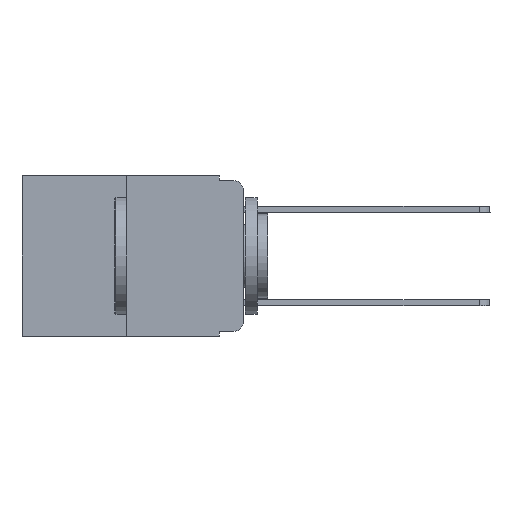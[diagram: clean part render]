
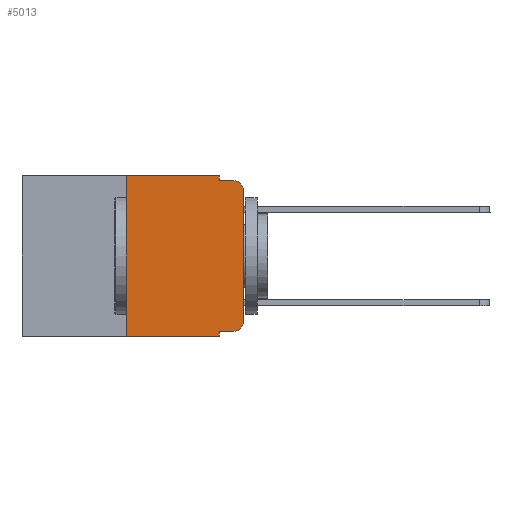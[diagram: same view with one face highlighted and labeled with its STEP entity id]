
A CAD part, left-side view. The second image highlights one B-rep face of the part: STEP entity #5013.
In plain terms, the highlighted planar face has unit normal (-1, 0, 0).
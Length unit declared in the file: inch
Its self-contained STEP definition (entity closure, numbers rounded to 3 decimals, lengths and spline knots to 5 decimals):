
#557 = VECTOR ( 'NONE', #19836, 39.37008 ) ;
#812 = VECTOR ( 'NONE', #2644, 39.37008 ) ;
#824 = VERTEX_POINT ( 'NONE', #6259 ) ;
#881 = EDGE_CURVE ( 'NONE', #18751, #15589, #11647, .T. ) ;
#998 = CARTESIAN_POINT ( 'NONE',  ( 0., 0.25, 0. ) ) ;
#1251 = PLANE ( 'NONE',  #21415 ) ;
#1456 = CARTESIAN_POINT ( 'NONE',  ( 0., 0.02, -0.333 ) ) ;
#1478 = EDGE_CURVE ( 'NONE', #9286, #5018, #22921, .T. ) ;
#2509 = ORIENTED_EDGE ( 'NONE', *, *, #4705, .F. ) ;
#2516 = ORIENTED_EDGE ( 'NONE', *, *, #18826, .T. ) ;
#2592 = CARTESIAN_POINT ( 'NONE',  ( 0., 0., -0.03 ) ) ;
#2644 = DIRECTION ( 'NONE',  ( 0., 0., 1. ) ) ;
#3015 = VECTOR ( 'NONE', #19449, 39.37008 ) ;
#3838 = VECTOR ( 'NONE', #9369, 39.37008 ) ;
#3944 = CARTESIAN_POINT ( 'NONE',  ( 0., 0.02, -0.01 ) ) ;
#4252 = VECTOR ( 'NONE', #14095, 39.37008 ) ;
#4310 = VECTOR ( 'NONE', #19058, 39.37008 ) ;
#4334 = CARTESIAN_POINT ( 'NONE',  ( 0., 0.051, -0.01 ) ) ;
#4543 = ORIENTED_EDGE ( 'NONE', *, *, #9656, .T. ) ;
#4638 = FACE_OUTER_BOUND ( 'NONE', #16369, .T. ) ;
#4705 = EDGE_CURVE ( 'NONE', #15589, #824, #17960, .T. ) ;
#4799 = DIRECTION ( 'NONE',  ( -1., 0., 0. ) ) ;
#4859 = VERTEX_POINT ( 'NONE', #7562 ) ;
#4934 = CARTESIAN_POINT ( 'NONE',  ( 0., 0.051, 0. ) ) ;
#5013 = ADVANCED_FACE ( 'NONE', ( #4638 ), #1251, .F. ) ;
#5018 = VERTEX_POINT ( 'NONE', #19012 ) ;
#5728 = CARTESIAN_POINT ( 'NONE',  ( 0., 0.051, -0.333 ) ) ;
#5732 = VECTOR ( 'NONE', #8753, 39.37008 ) ;
#6259 = CARTESIAN_POINT ( 'NONE',  ( 0., 0.051, 0. ) ) ;
#6827 = CARTESIAN_POINT ( 'NONE',  ( 0., 0.051, 0. ) ) ;
#7092 = CARTESIAN_POINT ( 'NONE',  ( 0., 0.473, 0. ) ) ;
#7562 = CARTESIAN_POINT ( 'NONE',  ( 0., 0., -0.313 ) ) ;
#7769 = ORIENTED_EDGE ( 'NONE', *, *, #881, .F. ) ;
#8027 = CARTESIAN_POINT ( 'NONE',  ( 0., 0.25, -0.343 ) ) ;
#8731 = ORIENTED_EDGE ( 'NONE', *, *, #15310, .F. ) ;
#8753 = DIRECTION ( 'NONE',  ( 0., -1., 0. ) ) ;
#8784 = ORIENTED_EDGE ( 'NONE', *, *, #20902, .T. ) ;
#9094 = DIRECTION ( 'NONE',  ( -1., 0., 0. ) ) ;
#9243 = VERTEX_POINT ( 'NONE', #4334 ) ;
#9258 = LINE ( 'NONE', #13116, #3838 ) ;
#9286 = VERTEX_POINT ( 'NONE', #5728 ) ;
#9369 = DIRECTION ( 'NONE',  ( 0., -1., 0. ) ) ;
#9451 = EDGE_CURVE ( 'NONE', #16069, #18055, #21424, .T. ) ;
#9656 = EDGE_CURVE ( 'NONE', #4859, #16069, #16575, .T. ) ;
#10129 = DIRECTION ( 'NONE',  ( 1., 0., 0. ) ) ;
#11147 = EDGE_CURVE ( 'NONE', #15769, #4859, #11750, .T. ) ;
#11474 = ORIENTED_EDGE ( 'NONE', *, *, #19363, .F. ) ;
#11647 = LINE ( 'NONE', #20402, #812 ) ;
#11750 = CIRCLE ( 'NONE', #13612, 0.02 ) ;
#11944 = DIRECTION ( 'NONE',  ( 0., 0., -1. ) ) ;
#12233 = LINE ( 'NONE', #6827, #3015 ) ;
#12729 = CARTESIAN_POINT ( 'NONE',  ( 0., 0.02, -0.313 ) ) ;
#13116 = CARTESIAN_POINT ( 'NONE',  ( 0., 0.051, -0.01 ) ) ;
#13612 = AXIS2_PLACEMENT_3D ( 'NONE', #12729, #9094, #21709 ) ;
#13970 = CARTESIAN_POINT ( 'NONE',  ( 0., 0.473, -0.343 ) ) ;
#14095 = DIRECTION ( 'NONE',  ( 0., -1., 0. ) ) ;
#14204 = LINE ( 'NONE', #13970, #4252 ) ;
#14818 = ORIENTED_EDGE ( 'NONE', *, *, #9451, .T. ) ;
#14901 = ORIENTED_EDGE ( 'NONE', *, *, #1478, .F. ) ;
#15310 = EDGE_CURVE ( 'NONE', #824, #9243, #12233, .T. ) ;
#15589 = VERTEX_POINT ( 'NONE', #998 ) ;
#15769 = VERTEX_POINT ( 'NONE', #1456 ) ;
#16069 = VERTEX_POINT ( 'NONE', #2592 ) ;
#16269 = LINE ( 'NONE', #16955, #4310 ) ;
#16369 = EDGE_LOOP ( 'NONE', ( #4543, #14818, #11474, #8731, #2509, #7769, #2516, #14901, #8784, #20721 ) ) ;
#16575 = LINE ( 'NONE', #18450, #557 ) ;
#16955 = CARTESIAN_POINT ( 'NONE',  ( 0., 0.051, -0.333 ) ) ;
#17379 = CARTESIAN_POINT ( 'NONE',  ( 0., 0.473, 0. ) ) ;
#17446 = DIRECTION ( 'NONE',  ( 0., 0., -1. ) ) ;
#17960 = LINE ( 'NONE', #7092, #5732 ) ;
#18055 = VERTEX_POINT ( 'NONE', #3944 ) ;
#18450 = CARTESIAN_POINT ( 'NONE',  ( 0., 0., 0. ) ) ;
#18751 = VERTEX_POINT ( 'NONE', #8027 ) ;
#18826 = EDGE_CURVE ( 'NONE', #18751, #5018, #14204, .T. ) ;
#18849 = VECTOR ( 'NONE', #17446, 39.37008 ) ;
#19012 = CARTESIAN_POINT ( 'NONE',  ( 0., 0.051, -0.343 ) ) ;
#19058 = DIRECTION ( 'NONE',  ( 0., -1., 0. ) ) ;
#19363 = EDGE_CURVE ( 'NONE', #9243, #18055, #9258, .T. ) ;
#19449 = DIRECTION ( 'NONE',  ( 0., 0., -1. ) ) ;
#19836 = DIRECTION ( 'NONE',  ( 0., 0., 1. ) ) ;
#20402 = CARTESIAN_POINT ( 'NONE',  ( 0., 0.25, 0. ) ) ;
#20721 = ORIENTED_EDGE ( 'NONE', *, *, #11147, .T. ) ;
#20770 = DIRECTION ( 'NONE',  ( 0., 0., -1. ) ) ;
#20808 = CARTESIAN_POINT ( 'NONE',  ( 0., 0.02, -0.03 ) ) ;
#20902 = EDGE_CURVE ( 'NONE', #9286, #15769, #16269, .T. ) ;
#21415 = AXIS2_PLACEMENT_3D ( 'NONE', #17379, #10129, #20770 ) ;
#21424 = CIRCLE ( 'NONE', #22923, 0.02 ) ;
#21709 = DIRECTION ( 'NONE',  ( 0., 0., -1. ) ) ;
#22921 = LINE ( 'NONE', #4934, #18849 ) ;
#22923 = AXIS2_PLACEMENT_3D ( 'NONE', #20808, #4799, #11944 ) ;
